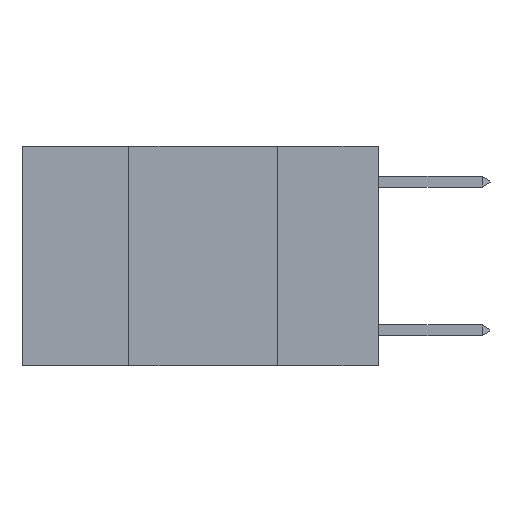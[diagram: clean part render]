
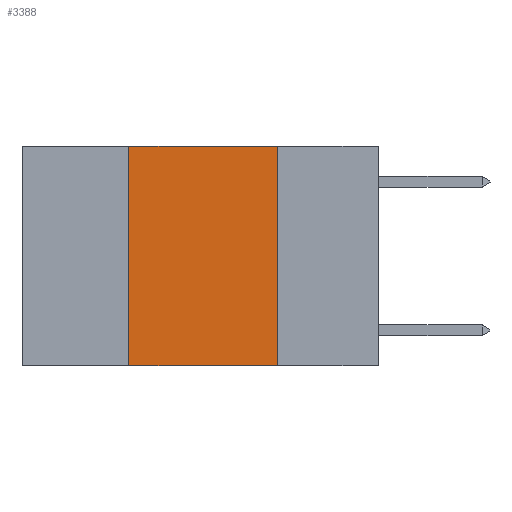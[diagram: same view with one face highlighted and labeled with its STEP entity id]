
A CAD part, left-side view. The second image highlights one B-rep face of the part: STEP entity #3388.
In plain terms, the highlighted planar face has unit normal (-1, 0, 0).
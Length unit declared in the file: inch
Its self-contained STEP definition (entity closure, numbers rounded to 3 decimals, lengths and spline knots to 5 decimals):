
#65 = ORIENTED_EDGE ( 'NONE', *, *, #5744, .F. ) ;
#506 = CARTESIAN_POINT ( 'NONE',  ( 0., 0.6, 0. ) ) ;
#784 = CARTESIAN_POINT ( 'NONE',  ( 0., 0.17, 0. ) ) ;
#1000 = LINE ( 'NONE', #9919, #3579 ) ;
#1799 = VECTOR ( 'NONE', #8726, 39.37008 ) ;
#1857 = CARTESIAN_POINT ( 'NONE',  ( 0., 0.6, 0. ) ) ;
#2733 = DIRECTION ( 'NONE',  ( 0., 0., -1. ) ) ;
#3388 = ADVANCED_FACE ( 'NONE', ( #6751 ), #9732, .F. ) ;
#3579 = VECTOR ( 'NONE', #4610, 39.37008 ) ;
#3741 = EDGE_CURVE ( 'NONE', #7733, #5619, #8348, .T. ) ;
#4033 = CARTESIAN_POINT ( 'NONE',  ( 0., 0.42, 0. ) ) ;
#4139 = ORIENTED_EDGE ( 'NONE', *, *, #3741, .F. ) ;
#4253 = EDGE_CURVE ( 'NONE', #8881, #7733, #1000, .T. ) ;
#4490 = EDGE_CURVE ( 'NONE', #8881, #5571, #10855, .T. ) ;
#4610 = DIRECTION ( 'NONE',  ( 0., 0., 1. ) ) ;
#5049 = CARTESIAN_POINT ( 'NONE',  ( 0., 0.6, -0.37 ) ) ;
#5114 = AXIS2_PLACEMENT_3D ( 'NONE', #1857, #8059, #2733 ) ;
#5571 = VERTEX_POINT ( 'NONE', #9835 ) ;
#5619 = VERTEX_POINT ( 'NONE', #9077 ) ;
#5744 = EDGE_CURVE ( 'NONE', #5619, #5571, #8836, .T. ) ;
#6259 = VECTOR ( 'NONE', #11155, 39.37008 ) ;
#6596 = VECTOR ( 'NONE', #9306, 39.37008 ) ;
#6751 = FACE_OUTER_BOUND ( 'NONE', #10319, .T. ) ;
#6994 = ORIENTED_EDGE ( 'NONE', *, *, #4490, .T. ) ;
#7079 = ORIENTED_EDGE ( 'NONE', *, *, #4253, .F. ) ;
#7733 = VERTEX_POINT ( 'NONE', #4033 ) ;
#8059 = DIRECTION ( 'NONE',  ( 1., 0., 0. ) ) ;
#8348 = LINE ( 'NONE', #506, #6596 ) ;
#8726 = DIRECTION ( 'NONE',  ( 0., 0., -1. ) ) ;
#8836 = LINE ( 'NONE', #784, #1799 ) ;
#8881 = VERTEX_POINT ( 'NONE', #10321 ) ;
#9077 = CARTESIAN_POINT ( 'NONE',  ( 0., 0.17, 0. ) ) ;
#9306 = DIRECTION ( 'NONE',  ( 0., -1., 0. ) ) ;
#9732 = PLANE ( 'NONE',  #5114 ) ;
#9835 = CARTESIAN_POINT ( 'NONE',  ( 0., 0.17, -0.37 ) ) ;
#9919 = CARTESIAN_POINT ( 'NONE',  ( 0., 0.42, 0. ) ) ;
#10319 = EDGE_LOOP ( 'NONE', ( #65, #4139, #7079, #6994 ) ) ;
#10321 = CARTESIAN_POINT ( 'NONE',  ( 0., 0.42, -0.37 ) ) ;
#10855 = LINE ( 'NONE', #5049, #6259 ) ;
#11155 = DIRECTION ( 'NONE',  ( 0., -1., 0. ) ) ;
